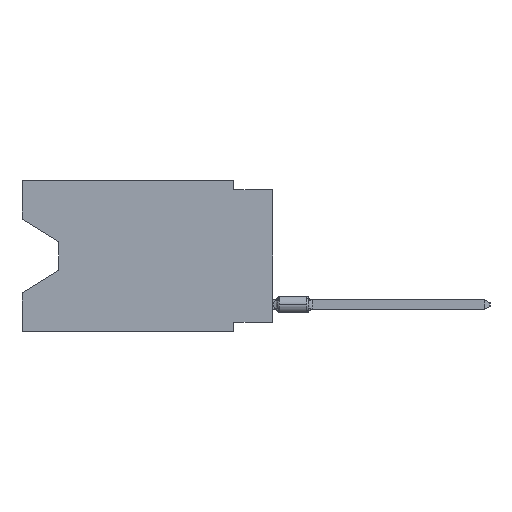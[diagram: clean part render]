
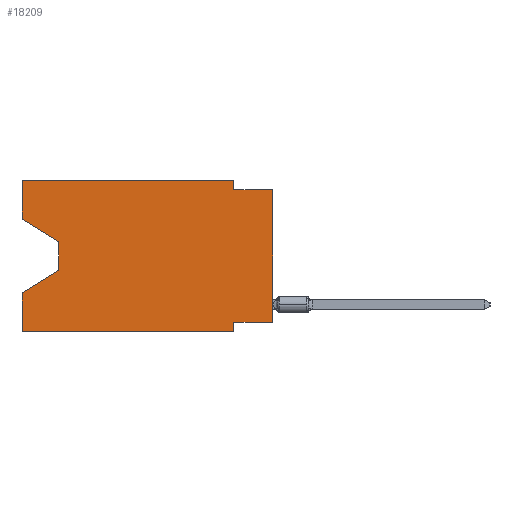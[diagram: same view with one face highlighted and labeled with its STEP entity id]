
A CAD part, left-side view. The second image highlights one B-rep face of the part: STEP entity #18209.
In plain terms, the highlighted planar face has unit normal (-1, 0, 0).
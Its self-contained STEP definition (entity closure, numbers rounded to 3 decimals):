
#24 = EDGE_CURVE ( 'NONE', #12756, #155, #24948, .T. ) ;
#155 = VERTEX_POINT ( 'NONE', #13776 ) ;
#687 = ORIENTED_EDGE ( 'NONE', *, *, #4770, .F. ) ;
#802 = CARTESIAN_POINT ( 'NONE',  ( 0., 16.383, -2.546 ) ) ;
#1084 = CARTESIAN_POINT ( 'NONE',  ( 0., 16.383, -2.546 ) ) ;
#1641 = VERTEX_POINT ( 'NONE', #28805 ) ;
#1774 = ORIENTED_EDGE ( 'NONE', *, *, #27654, .F. ) ;
#2573 = LINE ( 'NONE', #26528, #28857 ) ;
#2714 = DIRECTION ( 'NONE',  ( 1., 0., 0. ) ) ;
#2816 = DIRECTION ( 'NONE',  ( 0., 0., 1. ) ) ;
#3177 = LINE ( 'NONE', #15170, #20285 ) ;
#3538 = EDGE_CURVE ( 'NONE', #155, #11553, #13493, .T. ) ;
#3601 = LINE ( 'NONE', #12644, #36755 ) ;
#4770 = EDGE_CURVE ( 'NONE', #23175, #34088, #14534, .T. ) ;
#4881 = LINE ( 'NONE', #28456, #32475 ) ;
#5074 = DIRECTION ( 'NONE',  ( 0., -1., 0. ) ) ;
#5218 = EDGE_CURVE ( 'NONE', #12756, #38578, #3601, .T. ) ;
#5453 = ORIENTED_EDGE ( 'NONE', *, *, #8306, .T. ) ;
#6551 = EDGE_CURVE ( 'NONE', #34088, #38578, #4881, .T. ) ;
#7142 = EDGE_CURVE ( 'NONE', #1641, #18951, #11339, .T. ) ;
#7941 = ORIENTED_EDGE ( 'NONE', *, *, #21334, .T. ) ;
#8078 = VECTOR ( 'NONE', #15056, 1000. ) ;
#8306 = EDGE_CURVE ( 'NONE', #29147, #22478, #21632, .T. ) ;
#8571 = CARTESIAN_POINT ( 'NONE',  ( 0., 2.54, -0.635 ) ) ;
#8843 = VECTOR ( 'NONE', #34467, 1000. ) ;
#9253 = DIRECTION ( 'NONE',  ( 0., -1., 0. ) ) ;
#11339 = LINE ( 'NONE', #38402, #22468 ) ;
#11553 = VERTEX_POINT ( 'NONE', #25338 ) ;
#11934 = LINE ( 'NONE', #35860, #20516 ) ;
#12045 = ORIENTED_EDGE ( 'NONE', *, *, #16941, .F. ) ;
#12304 = DIRECTION ( 'NONE',  ( 0., 0., -1. ) ) ;
#12644 = CARTESIAN_POINT ( 'NONE',  ( 0., 0., 0. ) ) ;
#12756 = VERTEX_POINT ( 'NONE', #14695 ) ;
#12953 = DIRECTION ( 'NONE',  ( 0., 0., 1. ) ) ;
#13493 = LINE ( 'NONE', #37432, #8078 ) ;
#13776 = CARTESIAN_POINT ( 'NONE',  ( 0., 2.54, -9.271 ) ) ;
#13946 = FACE_OUTER_BOUND ( 'NONE', #35432, .T. ) ;
#14531 = PLANE ( 'NONE',  #36246 ) ;
#14534 = LINE ( 'NONE', #26482, #37991 ) ;
#14695 = CARTESIAN_POINT ( 'NONE',  ( 0., 0., -9.271 ) ) ;
#14709 = ORIENTED_EDGE ( 'NONE', *, *, #3538, .F. ) ;
#14838 = EDGE_CURVE ( 'NONE', #22478, #1641, #19358, .T. ) ;
#15056 = DIRECTION ( 'NONE',  ( 0., 0., -1. ) ) ;
#15170 = CARTESIAN_POINT ( 'NONE',  ( 0., 16.383, 0. ) ) ;
#15895 = CARTESIAN_POINT ( 'NONE',  ( 0., 16.383, 0. ) ) ;
#16229 = ORIENTED_EDGE ( 'NONE', *, *, #14838, .T. ) ;
#16941 = EDGE_CURVE ( 'NONE', #29147, #29899, #11934, .T. ) ;
#17077 = CARTESIAN_POINT ( 'NONE',  ( 0., 16.383, 0. ) ) ;
#18142 = VECTOR ( 'NONE', #36737, 1000. ) ;
#18209 = ADVANCED_FACE ( 'NONE', ( #13946 ), #14531, .F. ) ;
#18879 = DIRECTION ( 'NONE',  ( 0., 1., 0. ) ) ;
#18951 = VERTEX_POINT ( 'NONE', #19922 ) ;
#19358 = LINE ( 'NONE', #22507, #8843 ) ;
#19922 = CARTESIAN_POINT ( 'NONE',  ( 0., 16.383, -7.36 ) ) ;
#20285 = VECTOR ( 'NONE', #9253, 1000. ) ;
#20346 = DIRECTION ( 'NONE',  ( 0., 0.855, -0.519 ) ) ;
#20456 = VECTOR ( 'NONE', #12953, 1000. ) ;
#20516 = VECTOR ( 'NONE', #29978, 1000. ) ;
#20714 = EDGE_CURVE ( 'NONE', #29899, #23175, #3177, .T. ) ;
#21028 = ORIENTED_EDGE ( 'NONE', *, *, #6551, .F. ) ;
#21334 = EDGE_CURVE ( 'NONE', #30400, #11553, #2573, .T. ) ;
#21632 = LINE ( 'NONE', #802, #18142 ) ;
#22468 = VECTOR ( 'NONE', #20346, 1000. ) ;
#22478 = VERTEX_POINT ( 'NONE', #23584 ) ;
#22507 = CARTESIAN_POINT ( 'NONE',  ( 0., 13.97, -4.013 ) ) ;
#23175 = VERTEX_POINT ( 'NONE', #30788 ) ;
#23584 = CARTESIAN_POINT ( 'NONE',  ( 0., 13.97, -4.013 ) ) ;
#23748 = DIRECTION ( 'NONE',  ( 0., 0., -1. ) ) ;
#24948 = LINE ( 'NONE', #33974, #38044 ) ;
#25338 = CARTESIAN_POINT ( 'NONE',  ( 0., 2.54, -9.906 ) ) ;
#26482 = CARTESIAN_POINT ( 'NONE',  ( 0., 2.54, 0. ) ) ;
#26528 = CARTESIAN_POINT ( 'NONE',  ( 0., 16.383, -9.906 ) ) ;
#26856 = ORIENTED_EDGE ( 'NONE', *, *, #7142, .T. ) ;
#27654 = EDGE_CURVE ( 'NONE', #30400, #18951, #33752, .T. ) ;
#28456 = CARTESIAN_POINT ( 'NONE',  ( 0., 0., -0.635 ) ) ;
#28574 = ORIENTED_EDGE ( 'NONE', *, *, #20714, .F. ) ;
#28626 = ORIENTED_EDGE ( 'NONE', *, *, #5218, .T. ) ;
#28805 = CARTESIAN_POINT ( 'NONE',  ( 0., 13.97, -5.893 ) ) ;
#28857 = VECTOR ( 'NONE', #38503, 1000. ) ;
#29147 = VERTEX_POINT ( 'NONE', #1084 ) ;
#29899 = VERTEX_POINT ( 'NONE', #37671 ) ;
#29978 = DIRECTION ( 'NONE',  ( 0., 0., 1. ) ) ;
#30400 = VERTEX_POINT ( 'NONE', #38778 ) ;
#30788 = CARTESIAN_POINT ( 'NONE',  ( 0., 2.54, 0. ) ) ;
#31594 = ORIENTED_EDGE ( 'NONE', *, *, #24, .F. ) ;
#32475 = VECTOR ( 'NONE', #5074, 1000. ) ;
#33752 = LINE ( 'NONE', #15895, #20456 ) ;
#33974 = CARTESIAN_POINT ( 'NONE',  ( 0., 0., -9.271 ) ) ;
#34088 = VERTEX_POINT ( 'NONE', #8571 ) ;
#34467 = DIRECTION ( 'NONE',  ( 0., 0., -1. ) ) ;
#35432 = EDGE_LOOP ( 'NONE', ( #5453, #16229, #26856, #1774, #7941, #14709, #31594, #28626, #21028, #687, #28574, #12045 ) ) ;
#35860 = CARTESIAN_POINT ( 'NONE',  ( 0., 16.383, 0. ) ) ;
#36094 = CARTESIAN_POINT ( 'NONE',  ( 0., 0., -0.635 ) ) ;
#36246 = AXIS2_PLACEMENT_3D ( 'NONE', #17077, #2714, #23748 ) ;
#36737 = DIRECTION ( 'NONE',  ( 0., -0.855, -0.519 ) ) ;
#36755 = VECTOR ( 'NONE', #2816, 1000. ) ;
#37432 = CARTESIAN_POINT ( 'NONE',  ( 0., 2.54, -9.906 ) ) ;
#37671 = CARTESIAN_POINT ( 'NONE',  ( 0., 16.383, 0. ) ) ;
#37991 = VECTOR ( 'NONE', #12304, 1000. ) ;
#38044 = VECTOR ( 'NONE', #18879, 1000. ) ;
#38402 = CARTESIAN_POINT ( 'NONE',  ( 0., 13.97, -5.893 ) ) ;
#38503 = DIRECTION ( 'NONE',  ( 0., -1., 0. ) ) ;
#38578 = VERTEX_POINT ( 'NONE', #36094 ) ;
#38778 = CARTESIAN_POINT ( 'NONE',  ( 0., 16.383, -9.906 ) ) ;
